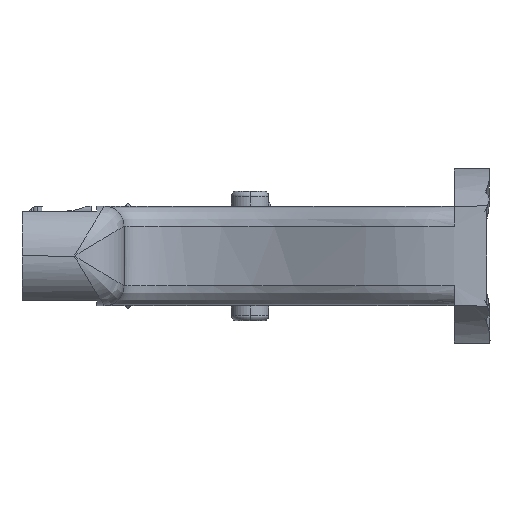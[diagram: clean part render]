
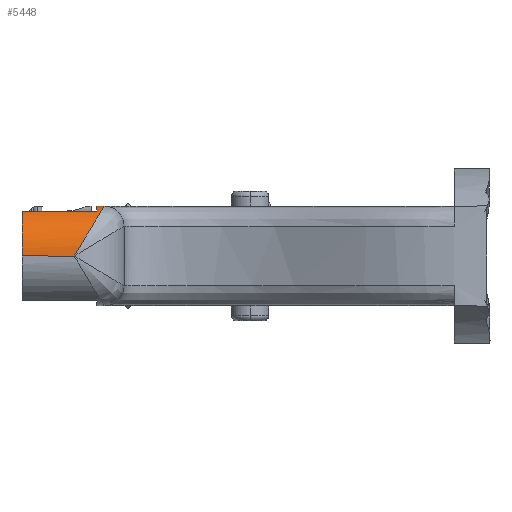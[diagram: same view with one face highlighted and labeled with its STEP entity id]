
A CAD part, left-side view. The second image highlights one B-rep face of the part: STEP entity #5448.
In plain terms, the highlighted cylindrical face has radius 10 mm (diameter 20 mm), a partial arc.
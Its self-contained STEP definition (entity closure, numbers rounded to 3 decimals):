
#34 = CARTESIAN_POINT ( 'NONE',  ( -89.359, 47.5, 26.5 ) ) ;
#426 = CARTESIAN_POINT ( 'NONE',  ( -95., 33.485, 23.358 ) ) ;
#1599 = CARTESIAN_POINT ( 'NONE',  ( -85., 31., 17.5 ) ) ;
#1688 = FACE_OUTER_BOUND ( 'NONE', #15461, .T. ) ;
#1808 = VECTOR ( 'NONE', #13040, 1000. ) ;
#2690 = LINE ( 'NONE', #7786, #10834 ) ;
#3495 = DIRECTION ( 'NONE',  ( 0., 0., 1. ) ) ;
#3939 = ORIENTED_EDGE ( 'NONE', *, *, #7688, .F. ) ;
#3959 = ORIENTED_EDGE ( 'NONE', *, *, #14823, .F. ) ;
#4652 = ORIENTED_EDGE ( 'NONE', *, *, #11027, .T. ) ;
#5382 = DIRECTION ( 'NONE',  ( 0., 1., 0. ) ) ;
#5448 = ADVANCED_FACE ( 'NONE', ( #1688 ), #8901, .T. ) ;
#5865 = AXIS2_PLACEMENT_3D ( 'NONE', #7868, #6658, #3495 ) ;
#5887 = DIRECTION ( 'NONE',  ( 0., -1., 0. ) ) ;
#5980 = VERTEX_POINT ( 'NONE', #14874 ) ;
#6251 = AXIS2_PLACEMENT_3D ( 'NONE', #10887, #13787, #13981 ) ;
#6658 = DIRECTION ( 'NONE',  ( 0., 1., 0. ) ) ;
#7249 = CARTESIAN_POINT ( 'NONE',  ( -95., 37., 17.5 ) ) ;
#7688 = EDGE_CURVE ( 'NONE', #10986, #18255, #17667, .T. ) ;
#7786 = CARTESIAN_POINT ( 'NONE',  ( -85., 31., 27.5 ) ) ;
#7868 = CARTESIAN_POINT ( 'NONE',  ( -85., 32.5, 17.5 ) ) ;
#8172 = LINE ( 'NONE', #14029, #18364 ) ;
#8882 = EDGE_CURVE ( 'NONE', #18255, #9252, #16736, .T. ) ;
#8901 = CYLINDRICAL_SURFACE ( 'NONE', #13328, 10. ) ;
#9205 = CARTESIAN_POINT ( 'NONE',  ( -90.858, 31., 27.5 ) ) ;
#9252 = VERTEX_POINT ( 'NONE', #9376 ) ;
#9376 = CARTESIAN_POINT ( 'NONE',  ( -89.359, 32.5, 26.5 ) ) ;
#10600 = CARTESIAN_POINT ( 'NONE',  ( -85., 31., 27.5 ) ) ;
#10834 = VECTOR ( 'NONE', #13377, 1000. ) ;
#10849 = CIRCLE ( 'NONE', #5865, 10. ) ;
#10887 = CARTESIAN_POINT ( 'NONE',  ( -85., 47.5, 17.5 ) ) ;
#10986 = VERTEX_POINT ( 'NONE', #11282 ) ;
#11027 = EDGE_CURVE ( 'NONE', #5980, #17881, #17173, .T. ) ;
#11282 = CARTESIAN_POINT ( 'NONE',  ( -95., 47.5, 17.5 ) ) ;
#11403 = ORIENTED_EDGE ( 'NONE', *, *, #13643, .F. ) ;
#11620 = DIRECTION ( 'NONE',  ( 0., 0., -1. ) ) ;
#11671 = VERTEX_POINT ( 'NONE', #14820 ) ;
#13040 = DIRECTION ( 'NONE',  ( 0., -1., 0. ) ) ;
#13328 = AXIS2_PLACEMENT_3D ( 'NONE', #1599, #5887, #11620 ) ;
#13377 = DIRECTION ( 'NONE',  ( 0., -1., 0. ) ) ;
#13634 = ORIENTED_EDGE ( 'NONE', *, *, #14449, .F. ) ;
#13643 = EDGE_CURVE ( 'NONE', #5980, #10986, #8172, .T. ) ;
#13787 = DIRECTION ( 'NONE',  ( 0., 1., 0. ) ) ;
#13981 = DIRECTION ( 'NONE',  ( 0., 0., -1. ) ) ;
#14029 = CARTESIAN_POINT ( 'NONE',  ( -95., 32.5, 17.5 ) ) ;
#14399 = CARTESIAN_POINT ( 'NONE',  ( -85., 31., 27.5 ) ) ;
#14449 = EDGE_CURVE ( 'NONE', #9252, #11671, #10849, .T. ) ;
#14820 = CARTESIAN_POINT ( 'NONE',  ( -85., 32.5, 27.5 ) ) ;
#14823 = EDGE_CURVE ( 'NONE', #11671, #17881, #2690, .T. ) ;
#14874 = CARTESIAN_POINT ( 'NONE',  ( -95., 37., 17.5 ) ) ;
#15461 = EDGE_LOOP ( 'NONE', ( #17656, #3939, #11403, #4652, #3959, #13634 ) ) ;
#16736 = LINE ( 'NONE', #34, #1808 ) ;
#17173 =( BOUNDED_CURVE ( )  B_SPLINE_CURVE ( 3, ( #7249, #426, #9205, #10600 ),
 .UNSPECIFIED., .F., .F. ) 
 B_SPLINE_CURVE_WITH_KNOTS ( ( 4, 4 ),
 ( 4.712, 6.283 ),
 .UNSPECIFIED. ) 
 CURVE ( )  GEOMETRIC_REPRESENTATION_ITEM ( )  RATIONAL_B_SPLINE_CURVE ( ( 1., 0.805, 0.805, 1. ) ) 
 REPRESENTATION_ITEM ( '' )  );
#17656 = ORIENTED_EDGE ( 'NONE', *, *, #8882, .F. ) ;
#17667 = CIRCLE ( 'NONE', #6251, 10. ) ;
#17881 = VERTEX_POINT ( 'NONE', #14399 ) ;
#18255 = VERTEX_POINT ( 'NONE', #18581 ) ;
#18364 = VECTOR ( 'NONE', #5382, 1000. ) ;
#18581 = CARTESIAN_POINT ( 'NONE',  ( -89.359, 47.5, 26.5 ) ) ;
